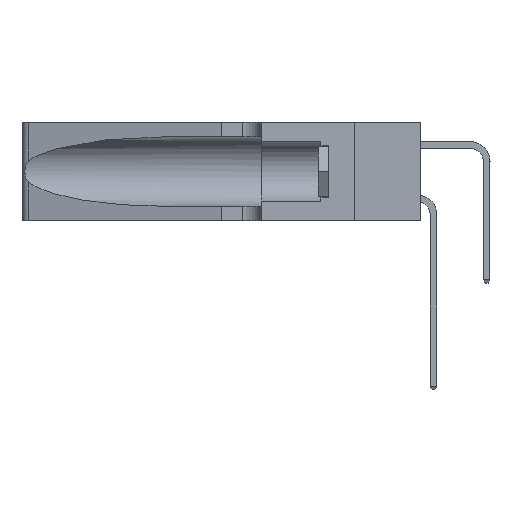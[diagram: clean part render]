
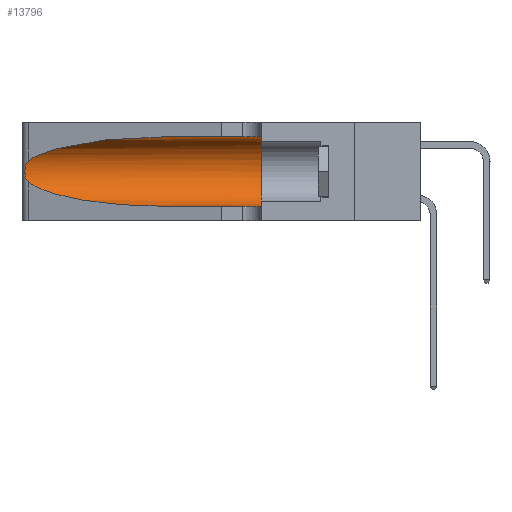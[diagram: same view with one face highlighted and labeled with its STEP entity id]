
A CAD part, left-side view. The second image highlights one B-rep face of the part: STEP entity #13796.
In plain terms, the highlighted cylindrical face has radius 3.308 mm (diameter 6.617 mm), a partial arc.
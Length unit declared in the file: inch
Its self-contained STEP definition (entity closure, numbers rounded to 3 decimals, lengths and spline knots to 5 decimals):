
#103 = CARTESIAN_POINT ( 'NONE',  ( 0.25487, 1.22718, 0.22369 ) ) ;
#153 = VERTEX_POINT ( 'NONE', #1797 ) ;
#344 = AXIS2_PLACEMENT_3D ( 'NONE', #567, #25442, #4164 ) ;
#400 = CARTESIAN_POINT ( 'NONE',  ( 0.25487, 1.22718, 0.14631 ) ) ;
#567 = CARTESIAN_POINT ( 'NONE',  ( 0.1305, 0.35, 0.185 ) ) ;
#1055 = DIRECTION ( 'NONE',  ( 0., 0., -1. ) ) ;
#1797 = CARTESIAN_POINT ( 'NONE',  ( 0.1305, 0.72297, 0.05475 ) ) ;
#3560 = CARTESIAN_POINT ( 'NONE',  ( 0.25856, 1.23593, 0.16098 ) ) ;
#4077 = CARTESIAN_POINT ( 'NONE',  ( 0.1305, 0.72297, 0.05475 ) ) ;
#4164 = DIRECTION ( 'NONE',  ( 0., 0., 1. ) ) ;
#4366 = ORIENTED_EDGE ( 'NONE', *, *, #44204, .T. ) ;
#5554 = CARTESIAN_POINT ( 'NONE',  ( 0.1305, 0.35, 0.31525 ) ) ;
#7015 = CARTESIAN_POINT ( 'NONE',  ( 0.25555, 1.22994, 0.2215 ) ) ;
#7163 = CARTESIAN_POINT ( 'NONE',  ( 0.25639, 1.23186, 0.15144 ) ) ;
#8612 = CYLINDRICAL_SURFACE ( 'NONE', #33589, 0.13025 ) ;
#9856 = VERTEX_POINT ( 'NONE', #400 ) ;
#10757 = CARTESIAN_POINT ( 'NONE',  ( 0.25487, 1.22718, 0.14631 ) ) ;
#10975 = ORIENTED_EDGE ( 'NONE', *, *, #12720, .F. ) ;
#11417 = EDGE_CURVE ( 'NONE', #153, #45748, #34794, .T. ) ;
#12219 = CARTESIAN_POINT ( 'NONE',  ( 0.26075, 1.23896, 0.178 ) ) ;
#12720 = EDGE_CURVE ( 'NONE', #42491, #40450, #15377, .T. ) ;
#13796 = ADVANCED_FACE ( 'NONE', ( #27463 ), #8612, .F. ) ;
#14178 = CARTESIAN_POINT ( 'NONE',  ( 0.25639, 1.23184, 0.21858 ) ) ;
#14314 = CARTESIAN_POINT ( 'NONE',  ( 0.1305, 0.72297, 0.31525 ) ) ;
#15377 = LINE ( 'NONE', #23725, #33059 ) ;
#15572 = CIRCLE ( 'NONE', #344, 0.13025 ) ;
#16542 = EDGE_CURVE ( 'NONE', #40450, #45748, #15572, .T. ) ;
#17150 = ORIENTED_EDGE ( 'NONE', *, *, #38131, .T. ) ;
#17707 =( BOUNDED_CURVE ( )  B_SPLINE_CURVE ( 3, ( #14314, #17850, #21442, #103 ),
 .UNSPECIFIED., .F., .F. ) 
 B_SPLINE_CURVE_WITH_KNOTS ( ( 4, 4 ),
 ( 1.5708, 2.84003 ),
 .UNSPECIFIED. ) 
 CURVE ( )  GEOMETRIC_REPRESENTATION_ITEM ( )  RATIONAL_B_SPLINE_CURVE ( ( 1., 0.87, 0.87, 1. ) ) 
 REPRESENTATION_ITEM ( '' )  );
#17716 = CARTESIAN_POINT ( 'NONE',  ( 0.25854, 1.2359, 0.20912 ) ) ;
#17850 = CARTESIAN_POINT ( 'NONE',  ( 0.18966, 0.96281, 0.31525 ) ) ;
#18078 = CARTESIAN_POINT ( 'NONE',  ( 0.25487, 1.22718, 0.14631 ) ) ;
#18222 = CARTESIAN_POINT ( 'NONE',  ( 0.2373, 1.15595, 0.08982 ) ) ;
#21304 = CARTESIAN_POINT ( 'NONE',  ( 0.26075, 1.23896, 0.19203 ) ) ;
#21442 = CARTESIAN_POINT ( 'NONE',  ( 0.2373, 1.15595, 0.28018 ) ) ;
#22383 = CARTESIAN_POINT ( 'NONE',  ( 0.1305, 1.61858, 0.185 ) ) ;
#22675 = CARTESIAN_POINT ( 'NONE',  ( 0.25487, 1.22718, 0.22369 ) ) ;
#23193 = CARTESIAN_POINT ( 'NONE',  ( 0.1305, 1.61858, 0.05475 ) ) ;
#23445 = CARTESIAN_POINT ( 'NONE',  ( 0.1305, 0.72297, 0.31525 ) ) ;
#23725 = CARTESIAN_POINT ( 'NONE',  ( 0.1305, 1.61858, 0.31525 ) ) ;
#24855 = CARTESIAN_POINT ( 'NONE',  ( 0.26017, 1.23833, 0.17102 ) ) ;
#25359 = CARTESIAN_POINT ( 'NONE',  ( 0.18966, 0.96281, 0.05475 ) ) ;
#25442 = DIRECTION ( 'NONE',  ( 0., 1., 0. ) ) ;
#27254 = DIRECTION ( 'NONE',  ( 0., -1., 0. ) ) ;
#27463 = FACE_OUTER_BOUND ( 'NONE', #33307, .T. ) ;
#28028 = VERTEX_POINT ( 'NONE', #22675 ) ;
#28414 = CARTESIAN_POINT ( 'NONE',  ( 0.25789, 1.23486, 0.15765 ) ) ;
#29326 = DIRECTION ( 'NONE',  ( 0., -1., 0. ) ) ;
#30757 = B_SPLINE_CURVE_WITH_KNOTS ( 'NONE', 3,
 ( #31775, #7015, #14178, #38886, #17716, #42437, #21304, #12219, #24855, #3560, #28414, #7163, #31933, #10757 ),
 .UNSPECIFIED., .F., .F.,
 ( 4, 2, 2, 2, 2, 2, 4 ),
 ( 0., 0.00027, 0.00053, 0.00107, 0.0016, 0.00187, 0.00214 ),
 .UNSPECIFIED. ) ;
#31775 = CARTESIAN_POINT ( 'NONE',  ( 0.25487, 1.22718, 0.22369 ) ) ;
#31933 = CARTESIAN_POINT ( 'NONE',  ( 0.25555, 1.22993, 0.14849 ) ) ;
#33059 = VECTOR ( 'NONE', #27254, 39.37008 ) ;
#33307 = EDGE_LOOP ( 'NONE', ( #17150, #42733, #4366, #43540, #38507, #10975 ) ) ;
#33589 = AXIS2_PLACEMENT_3D ( 'NONE', #22383, #29326, #1055 ) ;
#34794 = LINE ( 'NONE', #23193, #37013 ) ;
#36964 = CARTESIAN_POINT ( 'NONE',  ( 0.1305, 0.35, 0.05475 ) ) ;
#37013 = VECTOR ( 'NONE', #37222, 39.37008 ) ;
#37222 = DIRECTION ( 'NONE',  ( 0., -1., 0. ) ) ;
#38131 = EDGE_CURVE ( 'NONE', #42491, #28028, #17707, .T. ) ;
#38507 = ORIENTED_EDGE ( 'NONE', *, *, #16542, .F. ) ;
#38886 = CARTESIAN_POINT ( 'NONE',  ( 0.25787, 1.23484, 0.2124 ) ) ;
#38960 =( BOUNDED_CURVE ( )  B_SPLINE_CURVE ( 3, ( #18078, #18222, #25359, #4077 ),
 .UNSPECIFIED., .F., .T. ) 
 B_SPLINE_CURVE_WITH_KNOTS ( ( 4, 4 ),
 ( 3.44316, 4.71239 ),
 .UNSPECIFIED. ) 
 CURVE ( )  GEOMETRIC_REPRESENTATION_ITEM ( )  RATIONAL_B_SPLINE_CURVE ( ( 1., 0.87, 0.87, 1. ) ) 
 REPRESENTATION_ITEM ( '' )  );
#40450 = VERTEX_POINT ( 'NONE', #5554 ) ;
#42437 = CARTESIAN_POINT ( 'NONE',  ( 0.26018, 1.23835, 0.19895 ) ) ;
#42491 = VERTEX_POINT ( 'NONE', #23445 ) ;
#42733 = ORIENTED_EDGE ( 'NONE', *, *, #44788, .T. ) ;
#43540 = ORIENTED_EDGE ( 'NONE', *, *, #11417, .T. ) ;
#44204 = EDGE_CURVE ( 'NONE', #9856, #153, #38960, .T. ) ;
#44788 = EDGE_CURVE ( 'NONE', #28028, #9856, #30757, .T. ) ;
#45748 = VERTEX_POINT ( 'NONE', #36964 ) ;
